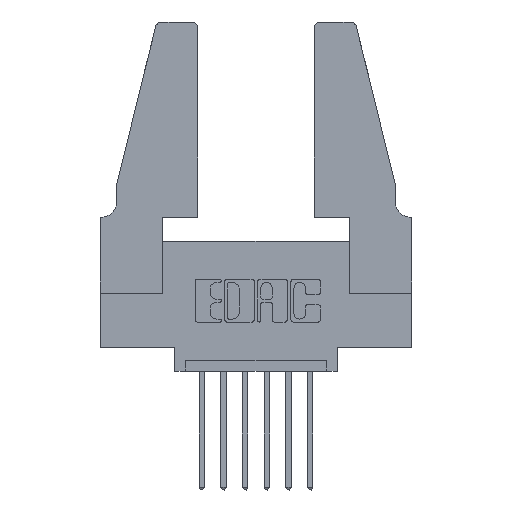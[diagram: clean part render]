
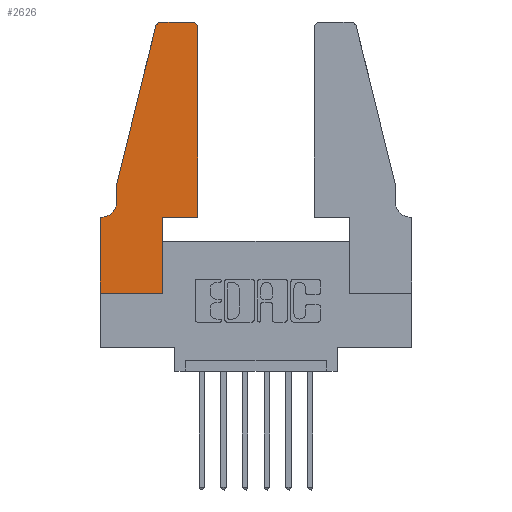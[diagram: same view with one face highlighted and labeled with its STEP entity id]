
A CAD part, top view. The second image highlights one B-rep face of the part: STEP entity #2626.
In plain terms, the highlighted planar face has unit normal (0, 0, 1).
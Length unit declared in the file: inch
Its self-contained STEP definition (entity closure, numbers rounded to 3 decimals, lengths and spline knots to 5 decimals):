
#133 = EDGE_CURVE ( 'NONE', #6116, #2240, #3690, .T. ) ;
#166 = ORIENTED_EDGE ( 'NONE', *, *, #4429, .T. ) ;
#169 = DIRECTION ( 'NONE',  ( -1., 0., 0. ) ) ;
#183 = EDGE_CURVE ( 'NONE', #9302, #1948, #1278, .T. ) ;
#284 = CARTESIAN_POINT ( 'NONE',  ( 0.284, 1.25, 0.37 ) ) ;
#303 = VERTEX_POINT ( 'NONE', #6364 ) ;
#325 = EDGE_LOOP ( 'NONE', ( #166, #2047, #4055, #1642, #11080, #5919, #1724, #5834, #2908, #6909, #6250, #9477 ) ) ;
#419 = LINE ( 'NONE', #2507, #9309 ) ;
#525 = EDGE_CURVE ( 'NONE', #2240, #9482, #419, .T. ) ;
#680 = DIRECTION ( 'NONE',  ( 0., 0., 1. ) ) ;
#708 = DIRECTION ( 'NONE',  ( 0., -1., 0. ) ) ;
#718 = DIRECTION ( 'NONE',  ( -0.239, -0.971, 0. ) ) ;
#1081 = DIRECTION ( 'NONE',  ( 1., 0., 0. ) ) ;
#1089 = AXIS2_PLACEMENT_3D ( 'NONE', #8089, #1723, #7998 ) ;
#1150 = VERTEX_POINT ( 'NONE', #6130 ) ;
#1208 = CARTESIAN_POINT ( 'NONE',  ( 0.0755, 0.5, 0.37 ) ) ;
#1278 = LINE ( 'NONE', #6251, #7497 ) ;
#1342 = AXIS2_PLACEMENT_3D ( 'NONE', #11480, #680, #7019 ) ;
#1471 = EDGE_CURVE ( 'NONE', #11121, #9302, #10427, .T. ) ;
#1564 = CARTESIAN_POINT ( 'NONE',  ( 0.2865, 0.35, 0.37 ) ) ;
#1591 = EDGE_CURVE ( 'NONE', #2234, #6116, #11543, .T. ) ;
#1606 = EDGE_CURVE ( 'NONE', #9482, #303, #5941, .T. ) ;
#1642 = ORIENTED_EDGE ( 'NONE', *, *, #525, .T. ) ;
#1723 = DIRECTION ( 'NONE',  ( 0., 0., -1. ) ) ;
#1724 = ORIENTED_EDGE ( 'NONE', *, *, #1471, .T. ) ;
#1887 = CARTESIAN_POINT ( 'NONE',  ( 0.4505, 0.35, 0.37 ) ) ;
#1948 = VERTEX_POINT ( 'NONE', #9496 ) ;
#2047 = ORIENTED_EDGE ( 'NONE', *, *, #1591, .T. ) ;
#2053 = DIRECTION ( 'NONE',  ( 0., 1., 0. ) ) ;
#2056 = LINE ( 'NONE', #1887, #10775 ) ;
#2234 = VERTEX_POINT ( 'NONE', #284 ) ;
#2240 = VERTEX_POINT ( 'NONE', #1208 ) ;
#2507 = CARTESIAN_POINT ( 'NONE',  ( 0.0755, 0.5, 0.37 ) ) ;
#2625 = CARTESIAN_POINT ( 'NONE',  ( 0.2865, 0.35, 0.37 ) ) ;
#2626 = ADVANCED_FACE ( 'NONE', ( #4614 ), #5189, .T. ) ;
#2647 = CARTESIAN_POINT ( 'NONE',  ( 0.284, 1.22, 0.37 ) ) ;
#2767 = DIRECTION ( 'NONE',  ( 1., 0., 0. ) ) ;
#2893 = LINE ( 'NONE', #5083, #10216 ) ;
#2908 = ORIENTED_EDGE ( 'NONE', *, *, #6056, .T. ) ;
#2919 = CARTESIAN_POINT ( 'NONE',  ( 0., 0.35, 0.37 ) ) ;
#3097 = VERTEX_POINT ( 'NONE', #2625 ) ;
#3448 = CARTESIAN_POINT ( 'NONE',  ( 0.4205, 1.25, 0.37 ) ) ;
#3462 = DIRECTION ( 'NONE',  ( 1., 0., 0. ) ) ;
#3555 = VECTOR ( 'NONE', #718, 39.37008 ) ;
#3687 = VECTOR ( 'NONE', #1081, 39.37008 ) ;
#3690 = LINE ( 'NONE', #4431, #3555 ) ;
#3814 = EDGE_CURVE ( 'NONE', #1150, #5109, #2056, .T. ) ;
#3870 = CARTESIAN_POINT ( 'NONE',  ( 0.0755, 0.35, 0.37 ) ) ;
#4020 = AXIS2_PLACEMENT_3D ( 'NONE', #11279, #9537, #7675 ) ;
#4055 = ORIENTED_EDGE ( 'NONE', *, *, #133, .T. ) ;
#4213 = EDGE_CURVE ( 'NONE', #303, #11121, #8829, .T. ) ;
#4214 = DIRECTION ( 'NONE',  ( -1., 0., 0. ) ) ;
#4429 = EDGE_CURVE ( 'NONE', #6337, #2234, #2893, .T. ) ;
#4431 = CARTESIAN_POINT ( 'NONE',  ( 0.0755, 0.5, 0.37 ) ) ;
#4614 = FACE_OUTER_BOUND ( 'NONE', #325, .T. ) ;
#5083 = CARTESIAN_POINT ( 'NONE',  ( 0.2605, 1.25, 0.37 ) ) ;
#5109 = VERTEX_POINT ( 'NONE', #7339 ) ;
#5189 = PLANE ( 'NONE',  #1342 ) ;
#5277 = DIRECTION ( 'NONE',  ( 0., -1., 0. ) ) ;
#5279 = AXIS2_PLACEMENT_3D ( 'NONE', #2647, #8151, #2767 ) ;
#5834 = ORIENTED_EDGE ( 'NONE', *, *, #183, .T. ) ;
#5871 = VECTOR ( 'NONE', #169, 39.37008 ) ;
#5919 = ORIENTED_EDGE ( 'NONE', *, *, #4213, .T. ) ;
#5941 = CIRCLE ( 'NONE', #1089, 0.07 ) ;
#6056 = EDGE_CURVE ( 'NONE', #1948, #3097, #6649, .T. ) ;
#6092 = LINE ( 'NONE', #6507, #3687 ) ;
#6116 = VERTEX_POINT ( 'NONE', #9142 ) ;
#6130 = CARTESIAN_POINT ( 'NONE',  ( 0.4505, 0.35, 0.37 ) ) ;
#6166 = EDGE_CURVE ( 'NONE', #5109, #6337, #9609, .T. ) ;
#6250 = ORIENTED_EDGE ( 'NONE', *, *, #3814, .T. ) ;
#6251 = CARTESIAN_POINT ( 'NONE',  ( 0., 0., 0.37 ) ) ;
#6337 = VERTEX_POINT ( 'NONE', #3448 ) ;
#6364 = CARTESIAN_POINT ( 'NONE',  ( 0.0055, 0.35, 0.37 ) ) ;
#6507 = CARTESIAN_POINT ( 'NONE',  ( 0.4505, 0.35, 0.37 ) ) ;
#6588 = CARTESIAN_POINT ( 'NONE',  ( 0., 0., 0.37 ) ) ;
#6589 = EDGE_CURVE ( 'NONE', #3097, #1150, #6092, .T. ) ;
#6649 = LINE ( 'NONE', #1564, #7772 ) ;
#6909 = ORIENTED_EDGE ( 'NONE', *, *, #6589, .T. ) ;
#7019 = DIRECTION ( 'NONE',  ( 1., 0., 0. ) ) ;
#7339 = CARTESIAN_POINT ( 'NONE',  ( 0.4505, 1.22, 0.37 ) ) ;
#7497 = VECTOR ( 'NONE', #3462, 39.37008 ) ;
#7675 = DIRECTION ( 'NONE',  ( 1., 0., 0. ) ) ;
#7772 = VECTOR ( 'NONE', #8723, 39.37008 ) ;
#7964 = CARTESIAN_POINT ( 'NONE',  ( 0., 0., 0.37 ) ) ;
#7998 = DIRECTION ( 'NONE',  ( -1., 0., 0. ) ) ;
#8089 = CARTESIAN_POINT ( 'NONE',  ( 0.0055, 0.42, 0.37 ) ) ;
#8151 = DIRECTION ( 'NONE',  ( 0., 0., 1. ) ) ;
#8723 = DIRECTION ( 'NONE',  ( 0., 1., 0. ) ) ;
#8774 = CARTESIAN_POINT ( 'NONE',  ( 0.0755, 0.42, 0.37 ) ) ;
#8829 = LINE ( 'NONE', #3870, #5871 ) ;
#9142 = CARTESIAN_POINT ( 'NONE',  ( 0.25487, 1.22718, 0.37 ) ) ;
#9302 = VERTEX_POINT ( 'NONE', #6588 ) ;
#9309 = VECTOR ( 'NONE', #5277, 39.37008 ) ;
#9477 = ORIENTED_EDGE ( 'NONE', *, *, #6166, .T. ) ;
#9482 = VERTEX_POINT ( 'NONE', #8774 ) ;
#9496 = CARTESIAN_POINT ( 'NONE',  ( 0.2865, 0., 0.37 ) ) ;
#9537 = DIRECTION ( 'NONE',  ( 0., 0., 1. ) ) ;
#9609 = CIRCLE ( 'NONE', #4020, 0.03 ) ;
#10216 = VECTOR ( 'NONE', #4214, 39.37008 ) ;
#10289 = VECTOR ( 'NONE', #708, 39.37008 ) ;
#10427 = LINE ( 'NONE', #7964, #10289 ) ;
#10775 = VECTOR ( 'NONE', #2053, 39.37008 ) ;
#11080 = ORIENTED_EDGE ( 'NONE', *, *, #1606, .T. ) ;
#11121 = VERTEX_POINT ( 'NONE', #2919 ) ;
#11279 = CARTESIAN_POINT ( 'NONE',  ( 0.4205, 1.22, 0.37 ) ) ;
#11480 = CARTESIAN_POINT ( 'NONE',  ( 0., 0.35, 0.37 ) ) ;
#11543 = CIRCLE ( 'NONE', #5279, 0.03 ) ;
